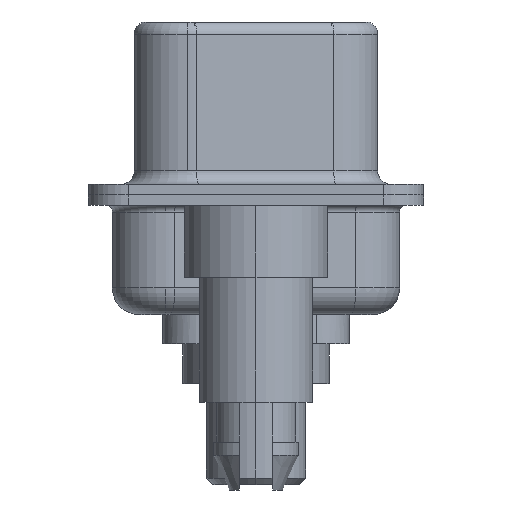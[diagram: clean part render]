
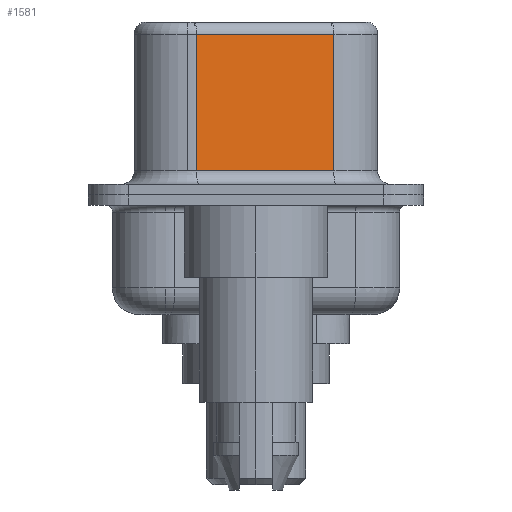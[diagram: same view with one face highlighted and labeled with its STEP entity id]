
A CAD part, left-side view. The second image highlights one B-rep face of the part: STEP entity #1581.
In plain terms, the highlighted planar face has unit normal (-0.985, -0.174, 0).
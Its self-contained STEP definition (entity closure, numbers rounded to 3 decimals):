
#21 = CARTESIAN_POINT ( 'NONE',  ( 4.58, -2.927, 6.02 ) ) ;
#720 = LINE ( 'NONE', #21, #5611 ) ;
#1210 = VERTEX_POINT ( 'NONE', #5309 ) ;
#1264 = AXIS2_PLACEMENT_3D ( 'NONE', #16381, #8493, #2139 ) ;
#1581 = ADVANCED_FACE ( 'NONE', ( #4061 ), #16552, .F. ) ;
#1724 = EDGE_LOOP ( 'NONE', ( #13946, #3808, #6626, #9611 ) ) ;
#1766 = VECTOR ( 'NONE', #8079, 1000. ) ;
#2139 = DIRECTION ( 'NONE',  ( -0.174, 0.985, 0. ) ) ;
#2716 = CARTESIAN_POINT ( 'NONE',  ( 4.58, -2.927, 0.9 ) ) ;
#3420 = LINE ( 'NONE', #15175, #15917 ) ;
#3457 = EDGE_CURVE ( 'NONE', #14795, #7135, #9119, .T. ) ;
#3808 = ORIENTED_EDGE ( 'NONE', *, *, #14534, .T. ) ;
#4061 = FACE_OUTER_BOUND ( 'NONE', #1724, .T. ) ;
#4819 = CARTESIAN_POINT ( 'NONE',  ( 4.58, -2.927, 6.52 ) ) ;
#4980 = CARTESIAN_POINT ( 'NONE',  ( 3.67, 2.233, 0.9 ) ) ;
#5309 = CARTESIAN_POINT ( 'NONE',  ( 3.67, 2.233, 6.02 ) ) ;
#5611 = VECTOR ( 'NONE', #8911, 1000. ) ;
#6626 = ORIENTED_EDGE ( 'NONE', *, *, #13935, .T. ) ;
#6736 = VECTOR ( 'NONE', #15398, 1000. ) ;
#6998 = EDGE_CURVE ( 'NONE', #16779, #7135, #12891, .T. ) ;
#7135 = VERTEX_POINT ( 'NONE', #2716 ) ;
#8079 = DIRECTION ( 'NONE',  ( 0.174, -0.985, 0. ) ) ;
#8493 = DIRECTION ( 'NONE',  ( 0.985, 0.174, 0. ) ) ;
#8911 = DIRECTION ( 'NONE',  ( -0.174, 0.985, 0. ) ) ;
#9119 = LINE ( 'NONE', #15788, #1766 ) ;
#9611 = ORIENTED_EDGE ( 'NONE', *, *, #3457, .T. ) ;
#10587 = CARTESIAN_POINT ( 'NONE',  ( 4.58, -2.927, 6.02 ) ) ;
#12603 = DIRECTION ( 'NONE',  ( 0., 0., -1. ) ) ;
#12891 = LINE ( 'NONE', #4819, #6736 ) ;
#13935 = EDGE_CURVE ( 'NONE', #1210, #14795, #3420, .T. ) ;
#13946 = ORIENTED_EDGE ( 'NONE', *, *, #6998, .F. ) ;
#14534 = EDGE_CURVE ( 'NONE', #16779, #1210, #720, .T. ) ;
#14795 = VERTEX_POINT ( 'NONE', #4980 ) ;
#15175 = CARTESIAN_POINT ( 'NONE',  ( 3.67, 2.233, 6.52 ) ) ;
#15398 = DIRECTION ( 'NONE',  ( 0., 0., -1. ) ) ;
#15788 = CARTESIAN_POINT ( 'NONE',  ( 4.58, -2.927, 0.9 ) ) ;
#15917 = VECTOR ( 'NONE', #12603, 1000. ) ;
#16381 = CARTESIAN_POINT ( 'NONE',  ( 4.58, -2.927, 6.52 ) ) ;
#16552 = PLANE ( 'NONE',  #1264 ) ;
#16779 = VERTEX_POINT ( 'NONE', #10587 ) ;
